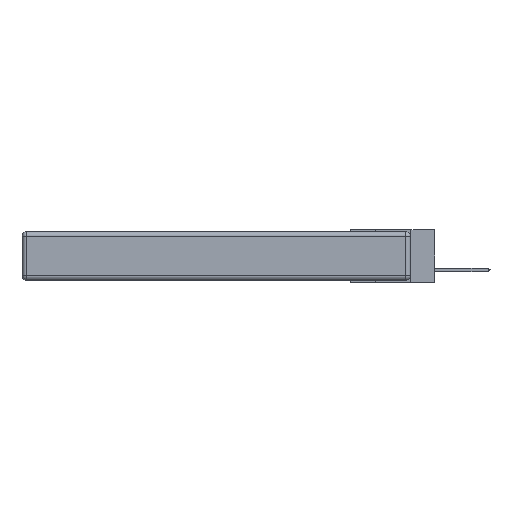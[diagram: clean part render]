
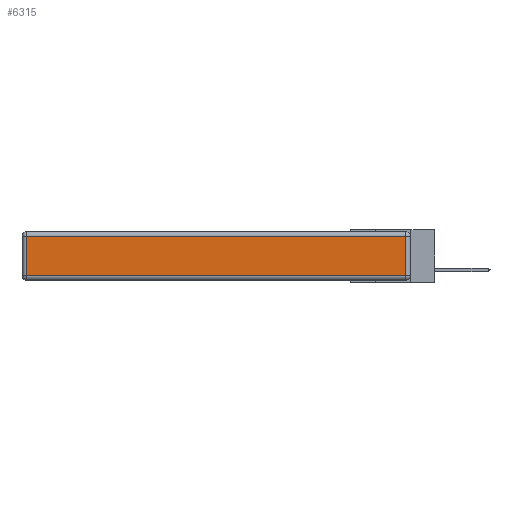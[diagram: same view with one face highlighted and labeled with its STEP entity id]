
A CAD part, left-side view. The second image highlights one B-rep face of the part: STEP entity #6315.
In plain terms, the highlighted planar face has unit normal (-1, 0, 0).
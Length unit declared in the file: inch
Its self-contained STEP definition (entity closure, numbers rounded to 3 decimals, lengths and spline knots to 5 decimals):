
#191 = ORIENTED_EDGE ( 'NONE', *, *, #6045, .T. ) ;
#629 = DIRECTION ( 'NONE',  ( 0., 0., 1. ) ) ;
#896 = CARTESIAN_POINT ( 'NONE',  ( 0., 2.72, -0.03 ) ) ;
#944 = EDGE_CURVE ( 'NONE', #2904, #12482, #12159, .T. ) ;
#1153 = CARTESIAN_POINT ( 'NONE',  ( 0., 0., -0.313 ) ) ;
#1880 = VECTOR ( 'NONE', #13353, 39.37008 ) ;
#1991 = EDGE_LOOP ( 'NONE', ( #2350, #7014, #12386, #191 ) ) ;
#2350 = ORIENTED_EDGE ( 'NONE', *, *, #944, .T. ) ;
#2737 = CARTESIAN_POINT ( 'NONE',  ( 0., 0., -0.343 ) ) ;
#2904 = VERTEX_POINT ( 'NONE', #6193 ) ;
#3616 = LINE ( 'NONE', #5880, #1880 ) ;
#4420 = FACE_OUTER_BOUND ( 'NONE', #1991, .T. ) ;
#4852 = CARTESIAN_POINT ( 'NONE',  ( 0., 0.03, -0.343 ) ) ;
#4955 = PLANE ( 'NONE',  #8535 ) ;
#4985 = VECTOR ( 'NONE', #9652, 39.37008 ) ;
#5503 = VERTEX_POINT ( 'NONE', #896 ) ;
#5880 = CARTESIAN_POINT ( 'NONE',  ( 0., 2.72, -0.343 ) ) ;
#5883 = VERTEX_POINT ( 'NONE', #11019 ) ;
#6045 = EDGE_CURVE ( 'NONE', #5503, #2904, #3616, .T. ) ;
#6193 = CARTESIAN_POINT ( 'NONE',  ( 0., 2.72, -0.313 ) ) ;
#6315 = ADVANCED_FACE ( 'NONE', ( #4420 ), #4955, .T. ) ;
#7014 = ORIENTED_EDGE ( 'NONE', *, *, #9788, .T. ) ;
#7590 = CARTESIAN_POINT ( 'NONE',  ( 0., 2.75, -0.03 ) ) ;
#8535 = AXIS2_PLACEMENT_3D ( 'NONE', #2737, #13535, #13356 ) ;
#8991 = CARTESIAN_POINT ( 'NONE',  ( 0., 0.03, -0.313 ) ) ;
#9652 = DIRECTION ( 'NONE',  ( 0., -1., 0. ) ) ;
#9788 = EDGE_CURVE ( 'NONE', #12482, #5883, #12844, .T. ) ;
#10422 = VECTOR ( 'NONE', #11782, 39.37008 ) ;
#10634 = VECTOR ( 'NONE', #629, 39.37008 ) ;
#11019 = CARTESIAN_POINT ( 'NONE',  ( 0., 0.03, -0.03 ) ) ;
#11374 = EDGE_CURVE ( 'NONE', #5883, #5503, #13633, .T. ) ;
#11782 = DIRECTION ( 'NONE',  ( 0., 1., 0. ) ) ;
#12159 = LINE ( 'NONE', #1153, #4985 ) ;
#12386 = ORIENTED_EDGE ( 'NONE', *, *, #11374, .T. ) ;
#12482 = VERTEX_POINT ( 'NONE', #8991 ) ;
#12844 = LINE ( 'NONE', #4852, #10634 ) ;
#13353 = DIRECTION ( 'NONE',  ( 0., 0., -1. ) ) ;
#13356 = DIRECTION ( 'NONE',  ( 0., 0., 1. ) ) ;
#13535 = DIRECTION ( 'NONE',  ( -1., 0., 0. ) ) ;
#13633 = LINE ( 'NONE', #7590, #10422 ) ;
